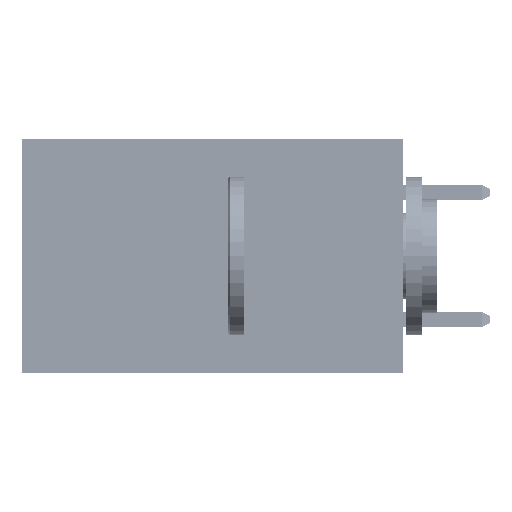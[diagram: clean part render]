
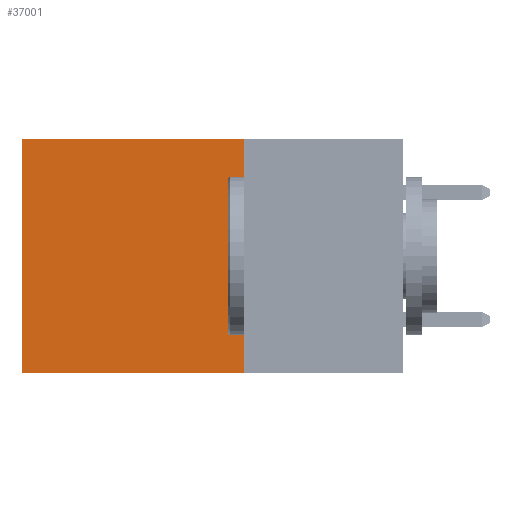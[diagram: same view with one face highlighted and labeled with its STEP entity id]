
A CAD part, left-side view. The second image highlights one B-rep face of the part: STEP entity #37001.
In plain terms, the highlighted planar face has unit normal (-1, 0, 0).
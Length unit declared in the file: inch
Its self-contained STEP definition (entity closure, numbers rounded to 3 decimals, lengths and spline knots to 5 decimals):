
#2301 = EDGE_CURVE ( 'NONE', #31796, #42523, #34810, .T. ) ;
#3137 = CARTESIAN_POINT ( 'NONE',  ( 0.2875, 0.25, -0.37 ) ) ;
#3842 = DIRECTION ( 'NONE',  ( 0., 0., -1. ) ) ;
#5540 = EDGE_CURVE ( 'NONE', #39280, #42523, #17822, .T. ) ;
#6588 = VECTOR ( 'NONE', #14880, 39.37008 ) ;
#7366 = ORIENTED_EDGE ( 'NONE', *, *, #2301, .F. ) ;
#9345 = CARTESIAN_POINT ( 'NONE',  ( 0.2875, 0.6, -0.37 ) ) ;
#9753 = CARTESIAN_POINT ( 'NONE',  ( 0.2875, 0.25, -0.37 ) ) ;
#11106 = CARTESIAN_POINT ( 'NONE',  ( 0.2875, 0.25, 0. ) ) ;
#13126 = LINE ( 'NONE', #40896, #27607 ) ;
#13973 = CARTESIAN_POINT ( 'NONE',  ( 0.2875, 0.25, 0. ) ) ;
#14052 = EDGE_CURVE ( 'NONE', #29600, #39280, #13126, .T. ) ;
#14880 = DIRECTION ( 'NONE',  ( 0., 0., -1. ) ) ;
#15321 = PLANE ( 'NONE',  #43834 ) ;
#17822 = LINE ( 'NONE', #32086, #48492 ) ;
#19693 = DIRECTION ( 'NONE',  ( 0., 1., 0. ) ) ;
#20411 = VECTOR ( 'NONE', #19693, 39.37008 ) ;
#20429 = ORIENTED_EDGE ( 'NONE', *, *, #14052, .T. ) ;
#20996 = ORIENTED_EDGE ( 'NONE', *, *, #5540, .T. ) ;
#21065 = ORIENTED_EDGE ( 'NONE', *, *, #47390, .F. ) ;
#23566 = FACE_OUTER_BOUND ( 'NONE', #43513, .T. ) ;
#27607 = VECTOR ( 'NONE', #41547, 39.37008 ) ;
#29600 = VERTEX_POINT ( 'NONE', #13973 ) ;
#31796 = VERTEX_POINT ( 'NONE', #3137 ) ;
#32086 = CARTESIAN_POINT ( 'NONE',  ( 0.2875, 0.6, 0. ) ) ;
#33113 = CARTESIAN_POINT ( 'NONE',  ( 0.2875, 0.6, 0. ) ) ;
#33874 = CARTESIAN_POINT ( 'NONE',  ( 0.2875, 0.25, 0. ) ) ;
#34810 = LINE ( 'NONE', #9753, #20411 ) ;
#36462 = DIRECTION ( 'NONE',  ( 0., 0., -1. ) ) ;
#37001 = ADVANCED_FACE ( 'NONE', ( #23566 ), #15321, .F. ) ;
#38587 = LINE ( 'NONE', #33874, #6588 ) ;
#39280 = VERTEX_POINT ( 'NONE', #33113 ) ;
#40896 = CARTESIAN_POINT ( 'NONE',  ( 0.2875, 0.25, 0. ) ) ;
#41547 = DIRECTION ( 'NONE',  ( 0., 1., 0. ) ) ;
#42523 = VERTEX_POINT ( 'NONE', #9345 ) ;
#43513 = EDGE_LOOP ( 'NONE', ( #20996, #7366, #21065, #20429 ) ) ;
#43834 = AXIS2_PLACEMENT_3D ( 'NONE', #11106, #46146, #3842 ) ;
#46146 = DIRECTION ( 'NONE',  ( 1., 0., 0. ) ) ;
#47390 = EDGE_CURVE ( 'NONE', #29600, #31796, #38587, .T. ) ;
#48492 = VECTOR ( 'NONE', #36462, 39.37008 ) ;
